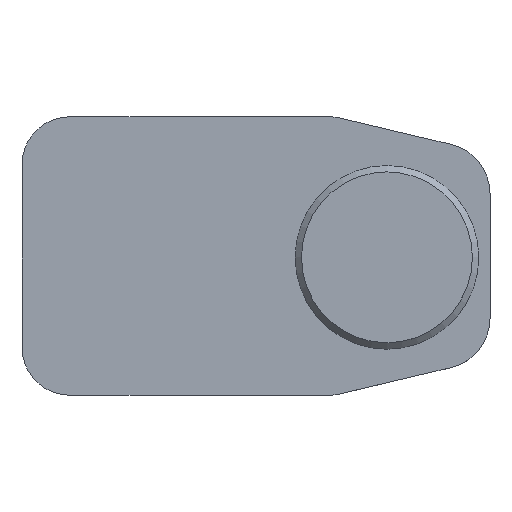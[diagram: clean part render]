
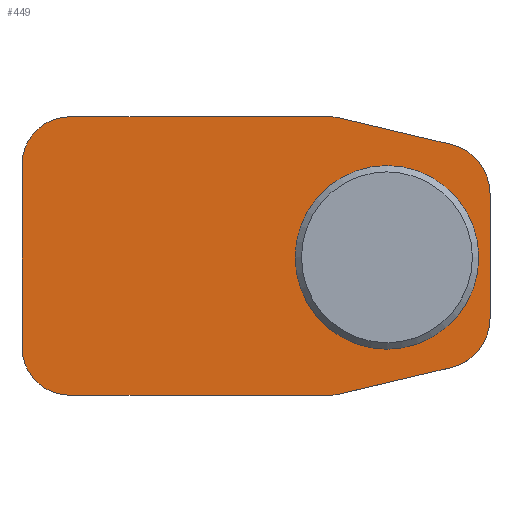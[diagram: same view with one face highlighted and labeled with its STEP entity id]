
A CAD part, top view. The second image highlights one B-rep face of the part: STEP entity #449.
In plain terms, the highlighted planar face has unit normal (0, 0, 1).
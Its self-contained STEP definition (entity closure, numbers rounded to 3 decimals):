
#15=FACE_BOUND('',#70,.T.);
#16=PLANE('',#495);
#40=FACE_OUTER_BOUND('',#69,.T.);
#69=EDGE_LOOP('',(#318,#319,#320,#321,#322,#323,#324,#325,#326,#327,#328,
#329));
#70=EDGE_LOOP('',(#330));
#99=LINE('',#702,#143);
#100=LINE('',#706,#144);
#101=LINE('',#710,#145);
#102=LINE('',#714,#146);
#103=LINE('',#718,#147);
#104=LINE('',#721,#148);
#143=VECTOR('',#558,10.);
#144=VECTOR('',#561,10.);
#145=VECTOR('',#564,10.);
#146=VECTOR('',#567,10.);
#147=VECTOR('',#570,10.);
#148=VECTOR('',#573,10.);
#185=CIRCLE('',#491,5.759);
#188=CIRCLE('',#496,3.);
#189=CIRCLE('',#497,2.675);
#190=CIRCLE('',#498,3.175);
#191=CIRCLE('',#499,3.175);
#192=CIRCLE('',#500,2.675);
#193=CIRCLE('',#501,3.);
#206=VERTEX_POINT('',#688);
#209=VERTEX_POINT('',#698);
#210=VERTEX_POINT('',#699);
#211=VERTEX_POINT('',#701);
#212=VERTEX_POINT('',#703);
#213=VERTEX_POINT('',#705);
#214=VERTEX_POINT('',#707);
#215=VERTEX_POINT('',#709);
#216=VERTEX_POINT('',#711);
#217=VERTEX_POINT('',#713);
#218=VERTEX_POINT('',#715);
#219=VERTEX_POINT('',#717);
#220=VERTEX_POINT('',#719);
#245=EDGE_CURVE('',#206,#206,#185,.T.);
#250=EDGE_CURVE('',#209,#210,#188,.T.);
#251=EDGE_CURVE('',#209,#211,#99,.F.);
#252=EDGE_CURVE('',#212,#211,#189,.T.);
#253=EDGE_CURVE('',#212,#213,#100,.F.);
#254=EDGE_CURVE('',#214,#213,#190,.T.);
#255=EDGE_CURVE('',#214,#215,#101,.T.);
#256=EDGE_CURVE('',#216,#215,#191,.T.);
#257=EDGE_CURVE('',#216,#217,#102,.F.);
#258=EDGE_CURVE('',#218,#217,#192,.T.);
#259=EDGE_CURVE('',#218,#219,#103,.F.);
#260=EDGE_CURVE('',#220,#219,#193,.T.);
#261=EDGE_CURVE('',#220,#210,#104,.T.);
#318=ORIENTED_EDGE('',*,*,#250,.F.);
#319=ORIENTED_EDGE('',*,*,#251,.T.);
#320=ORIENTED_EDGE('',*,*,#252,.F.);
#321=ORIENTED_EDGE('',*,*,#253,.T.);
#322=ORIENTED_EDGE('',*,*,#254,.F.);
#323=ORIENTED_EDGE('',*,*,#255,.T.);
#324=ORIENTED_EDGE('',*,*,#256,.F.);
#325=ORIENTED_EDGE('',*,*,#257,.T.);
#326=ORIENTED_EDGE('',*,*,#258,.F.);
#327=ORIENTED_EDGE('',*,*,#259,.T.);
#328=ORIENTED_EDGE('',*,*,#260,.F.);
#329=ORIENTED_EDGE('',*,*,#261,.T.);
#330=ORIENTED_EDGE('',*,*,#245,.F.);
#449=ADVANCED_FACE('',(#40,#15),#16,.T.);
#491=AXIS2_PLACEMENT_3D('',#689,#544,#545);
#495=AXIS2_PLACEMENT_3D('',#697,#554,#555);
#496=AXIS2_PLACEMENT_3D('',#700,#556,#557);
#497=AXIS2_PLACEMENT_3D('',#704,#559,#560);
#498=AXIS2_PLACEMENT_3D('',#708,#562,#563);
#499=AXIS2_PLACEMENT_3D('',#712,#565,#566);
#500=AXIS2_PLACEMENT_3D('',#716,#568,#569);
#501=AXIS2_PLACEMENT_3D('',#720,#571,#572);
#544=DIRECTION('center_axis',(0.,0.,1.));
#545=DIRECTION('ref_axis',(-1.,0.,0.));
#554=DIRECTION('center_axis',(0.,0.,1.));
#555=DIRECTION('ref_axis',(0.,-1.,0.));
#556=DIRECTION('center_axis',(0.,0.,-1.));
#557=DIRECTION('ref_axis',(-0.707,-0.707,0.));
#558=DIRECTION('',(-1.,0.,0.));
#559=DIRECTION('center_axis',(0.,0.,-1.));
#560=DIRECTION('ref_axis',(0.116,-0.993,0.));
#561=DIRECTION('',(-0.973,-0.231,0.));
#562=DIRECTION('center_axis',(0.,0.,-1.));
#563=DIRECTION('ref_axis',(0.785,-0.62,0.));
#564=DIRECTION('',(0.,1.,0.));
#565=DIRECTION('center_axis',(0.,0.,-1.));
#566=DIRECTION('ref_axis',(0.785,0.62,0.));
#567=DIRECTION('',(0.973,-0.231,0.));
#568=DIRECTION('center_axis',(0.,0.,-1.));
#569=DIRECTION('ref_axis',(0.116,0.993,0.));
#570=DIRECTION('',(1.,0.,0.));
#571=DIRECTION('center_axis',(0.,0.,-1.));
#572=DIRECTION('ref_axis',(-0.707,0.707,0.));
#573=DIRECTION('',(0.,-1.,0.));
#688=CARTESIAN_POINT('',(28.746,-0.089,1.651));
#689=CARTESIAN_POINT('Origin',(22.987,-0.089,1.651));
#697=CARTESIAN_POINT('Origin',(14.399,0.,1.651));
#698=CARTESIAN_POINT('',(3.095,-8.733,1.651));
#699=CARTESIAN_POINT('',(0.095,-5.733,1.651));
#700=CARTESIAN_POINT('Origin',(3.095,-5.733,1.651));
#701=CARTESIAN_POINT('',(19.39,-8.733,1.651));
#702=CARTESIAN_POINT('',(7.2,-8.733,1.651));
#703=CARTESIAN_POINT('',(20.007,-8.661,1.651));
#704=CARTESIAN_POINT('Origin',(19.39,-6.058,1.651));
#705=CARTESIAN_POINT('',(27.01,-6.998,1.651));
#706=CARTESIAN_POINT('',(18.145,-9.103,1.651));
#707=CARTESIAN_POINT('',(29.452,-3.909,1.651));
#708=CARTESIAN_POINT('Origin',(26.277,-3.909,1.651));
#709=CARTESIAN_POINT('',(29.452,3.909,1.651));
#710=CARTESIAN_POINT('',(29.452,-6.731,1.651));
#711=CARTESIAN_POINT('',(27.01,6.998,1.651));
#712=CARTESIAN_POINT('Origin',(26.277,3.909,1.651));
#713=CARTESIAN_POINT('',(20.007,8.661,1.651));
#714=CARTESIAN_POINT('',(23.415,7.852,1.651));
#715=CARTESIAN_POINT('',(19.39,8.733,1.651));
#716=CARTESIAN_POINT('Origin',(19.39,6.058,1.651));
#717=CARTESIAN_POINT('',(3.095,8.733,1.651));
#718=CARTESIAN_POINT('',(17.08,8.733,1.651));
#719=CARTESIAN_POINT('',(0.095,5.733,1.651));
#720=CARTESIAN_POINT('Origin',(3.095,5.733,1.651));
#721=CARTESIAN_POINT('',(0.095,4.616,1.651));
